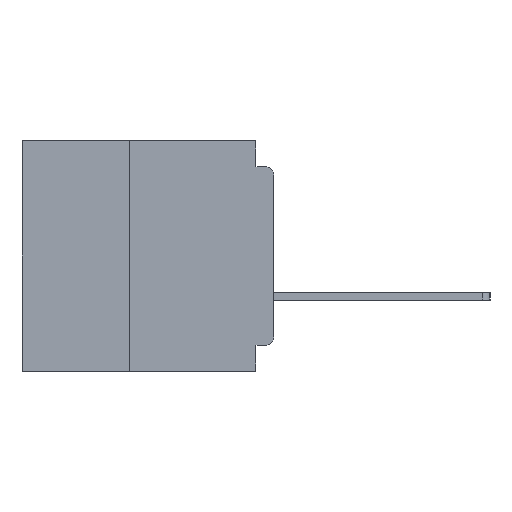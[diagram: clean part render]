
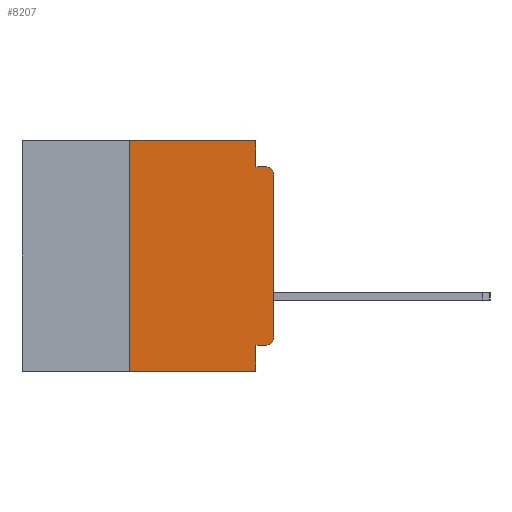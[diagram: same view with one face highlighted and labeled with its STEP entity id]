
A CAD part, left-side view. The second image highlights one B-rep face of the part: STEP entity #8207.
In plain terms, the highlighted planar face has unit normal (-1, 0, 0).
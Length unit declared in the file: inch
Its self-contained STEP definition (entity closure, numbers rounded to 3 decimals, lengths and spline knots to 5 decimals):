
#438 = CARTESIAN_POINT ( 'NONE',  ( 0., 0.031, -0.4 ) ) ;
#983 = DIRECTION ( 'NONE',  ( 0., 0., 1. ) ) ;
#1465 = LINE ( 'NONE', #19507, #38846 ) ;
#1970 = DIRECTION ( 'NONE',  ( -1., 0., 0. ) ) ;
#2022 = VECTOR ( 'NONE', #45865, 39.37008 ) ;
#2412 = VERTEX_POINT ( 'NONE', #438 ) ;
#2965 = LINE ( 'NONE', #23800, #41491 ) ;
#3555 = VERTEX_POINT ( 'NONE', #19180 ) ;
#4367 = ORIENTED_EDGE ( 'NONE', *, *, #5401, .F. ) ;
#4611 = CARTESIAN_POINT ( 'NONE',  ( 0., 0.25, -0.4 ) ) ;
#4953 = VECTOR ( 'NONE', #39845, 39.37008 ) ;
#5035 = VECTOR ( 'NONE', #44105, 39.37008 ) ;
#5401 = EDGE_CURVE ( 'NONE', #47324, #2412, #27228, .T. ) ;
#5703 = EDGE_CURVE ( 'NONE', #3555, #8135, #31819, .T. ) ;
#6148 = ORIENTED_EDGE ( 'NONE', *, *, #22020, .F. ) ;
#7350 = LINE ( 'NONE', #14252, #5035 ) ;
#7558 = CIRCLE ( 'NONE', #12876, 0.015 ) ;
#7644 = AXIS2_PLACEMENT_3D ( 'NONE', #33930, #37669, #15304 ) ;
#7768 = PLANE ( 'NONE',  #7644 ) ;
#8135 = VERTEX_POINT ( 'NONE', #14822 ) ;
#8207 = ADVANCED_FACE ( 'NONE', ( #46284 ), #7768, .F. ) ;
#10122 = VECTOR ( 'NONE', #983, 39.37008 ) ;
#11386 = VERTEX_POINT ( 'NONE', #31991 ) ;
#12876 = AXIS2_PLACEMENT_3D ( 'NONE', #24391, #1970, #28130 ) ;
#13310 = CARTESIAN_POINT ( 'NONE',  ( 0., 0.031, -0.355 ) ) ;
#13949 = ORIENTED_EDGE ( 'NONE', *, *, #23564, .F. ) ;
#14252 = CARTESIAN_POINT ( 'NONE',  ( 0., 0.437, -0.4 ) ) ;
#14822 = CARTESIAN_POINT ( 'NONE',  ( 0., 0.031, 0. ) ) ;
#14867 = LINE ( 'NONE', #17483, #4953 ) ;
#15304 = DIRECTION ( 'NONE',  ( 0., 0., -1. ) ) ;
#15409 = EDGE_CURVE ( 'NONE', #34194, #2412, #7350, .T. ) ;
#16056 = ORIENTED_EDGE ( 'NONE', *, *, #21729, .T. ) ;
#16361 = DIRECTION ( 'NONE',  ( 0., -1., 0. ) ) ;
#16512 = ORIENTED_EDGE ( 'NONE', *, *, #17909, .F. ) ;
#16733 = VERTEX_POINT ( 'NONE', #30530 ) ;
#17232 = VECTOR ( 'NONE', #29125, 39.37008 ) ;
#17483 = CARTESIAN_POINT ( 'NONE',  ( 0., 0., -0.355 ) ) ;
#17820 = CARTESIAN_POINT ( 'NONE',  ( 0., 0.031, -0.4 ) ) ;
#17909 = EDGE_CURVE ( 'NONE', #34194, #3555, #20096, .T. ) ;
#19180 = CARTESIAN_POINT ( 'NONE',  ( 0., 0.25, 0. ) ) ;
#19412 = VECTOR ( 'NONE', #16361, 39.37008 ) ;
#19507 = CARTESIAN_POINT ( 'NONE',  ( 0., 0., 0. ) ) ;
#19936 = ORIENTED_EDGE ( 'NONE', *, *, #27977, .F. ) ;
#20080 = CARTESIAN_POINT ( 'NONE',  ( 0., 0.015, -0.34 ) ) ;
#20085 = CARTESIAN_POINT ( 'NONE',  ( 0., 0.015, -0.045 ) ) ;
#20096 = LINE ( 'NONE', #41960, #10122 ) ;
#20133 = AXIS2_PLACEMENT_3D ( 'NONE', #20080, #46129, #23823 ) ;
#21729 = EDGE_CURVE ( 'NONE', #11386, #16733, #1465, .T. ) ;
#22020 = EDGE_CURVE ( 'NONE', #38180, #47324, #14867, .T. ) ;
#22922 = EDGE_CURVE ( 'NONE', #38180, #11386, #41036, .T. ) ;
#23564 = EDGE_CURVE ( 'NONE', #29403, #39619, #40391, .T. ) ;
#23575 = CARTESIAN_POINT ( 'NONE',  ( 0., 0.437, 0. ) ) ;
#23766 = CARTESIAN_POINT ( 'NONE',  ( 0., 0., -0.045 ) ) ;
#23800 = CARTESIAN_POINT ( 'NONE',  ( 0., 0.031, 0. ) ) ;
#23823 = DIRECTION ( 'NONE',  ( 0., 0., -1. ) ) ;
#24391 = CARTESIAN_POINT ( 'NONE',  ( 0., 0.015, -0.06 ) ) ;
#26068 = ORIENTED_EDGE ( 'NONE', *, *, #22922, .T. ) ;
#27228 = LINE ( 'NONE', #17820, #17232 ) ;
#27977 = EDGE_CURVE ( 'NONE', #8135, #29403, #2965, .T. ) ;
#28130 = DIRECTION ( 'NONE',  ( 0., 0., -1. ) ) ;
#28551 = CARTESIAN_POINT ( 'NONE',  ( 0., 0.031, -0.045 ) ) ;
#29125 = DIRECTION ( 'NONE',  ( 0., 0., -1. ) ) ;
#29403 = VERTEX_POINT ( 'NONE', #28551 ) ;
#29900 = ORIENTED_EDGE ( 'NONE', *, *, #5703, .F. ) ;
#30530 = CARTESIAN_POINT ( 'NONE',  ( 0., 0., -0.06 ) ) ;
#30760 = DIRECTION ( 'NONE',  ( 0., 0., 1. ) ) ;
#31819 = LINE ( 'NONE', #23575, #2022 ) ;
#31991 = CARTESIAN_POINT ( 'NONE',  ( 0., 0., -0.34 ) ) ;
#33000 = EDGE_LOOP ( 'NONE', ( #16056, #47595, #13949, #19936, #29900, #16512, #35285, #4367, #6148, #26068 ) ) ;
#33930 = CARTESIAN_POINT ( 'NONE',  ( 0., 0.437, 0. ) ) ;
#34194 = VERTEX_POINT ( 'NONE', #4611 ) ;
#35285 = ORIENTED_EDGE ( 'NONE', *, *, #15409, .T. ) ;
#37454 = CARTESIAN_POINT ( 'NONE',  ( 0., 0.015, -0.355 ) ) ;
#37669 = DIRECTION ( 'NONE',  ( 1., 0., 0. ) ) ;
#38180 = VERTEX_POINT ( 'NONE', #37454 ) ;
#38846 = VECTOR ( 'NONE', #30760, 39.37008 ) ;
#39619 = VERTEX_POINT ( 'NONE', #20085 ) ;
#39845 = DIRECTION ( 'NONE',  ( 0., 1., 0. ) ) ;
#40391 = LINE ( 'NONE', #23766, #19412 ) ;
#41036 = CIRCLE ( 'NONE', #20133, 0.015 ) ;
#41491 = VECTOR ( 'NONE', #46252, 39.37008 ) ;
#41960 = CARTESIAN_POINT ( 'NONE',  ( 0., 0.25, -0.4 ) ) ;
#44105 = DIRECTION ( 'NONE',  ( 0., -1., 0. ) ) ;
#45865 = DIRECTION ( 'NONE',  ( 0., -1., 0. ) ) ;
#46129 = DIRECTION ( 'NONE',  ( -1., 0., 0. ) ) ;
#46252 = DIRECTION ( 'NONE',  ( 0., 0., -1. ) ) ;
#46284 = FACE_OUTER_BOUND ( 'NONE', #33000, .T. ) ;
#47324 = VERTEX_POINT ( 'NONE', #13310 ) ;
#47595 = ORIENTED_EDGE ( 'NONE', *, *, #47855, .T. ) ;
#47855 = EDGE_CURVE ( 'NONE', #16733, #39619, #7558, .T. ) ;
